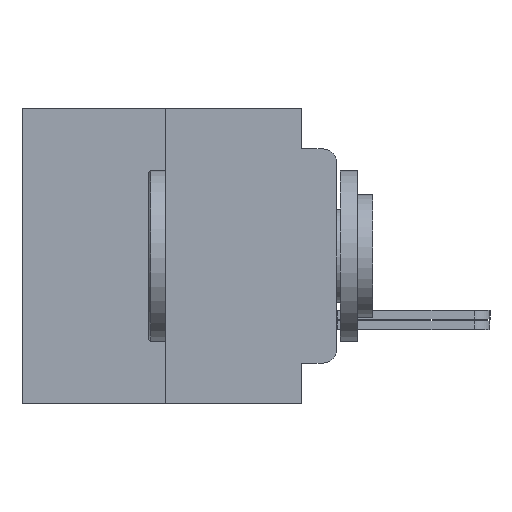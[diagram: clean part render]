
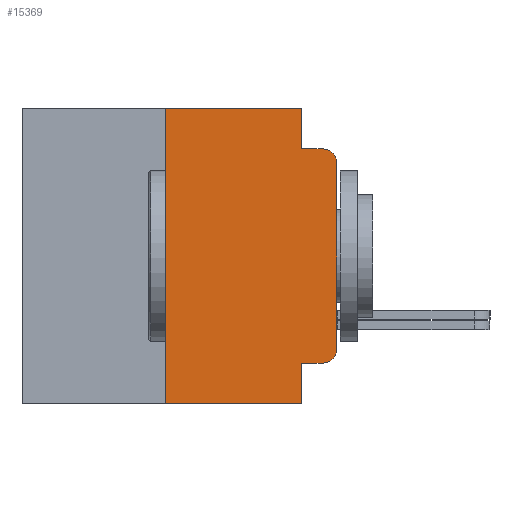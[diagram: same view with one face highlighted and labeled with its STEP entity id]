
A CAD part, left-side view. The second image highlights one B-rep face of the part: STEP entity #15369.
In plain terms, the highlighted planar face has unit normal (-1, 0, 0).
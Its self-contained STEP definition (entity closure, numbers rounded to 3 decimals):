
#266 = VERTEX_POINT ( 'NONE', #17163 ) ;
#475 = PLANE ( 'NONE',  #5160 ) ;
#850 = CARTESIAN_POINT ( 'NONE',  ( -75.603, 11.684, 5.486 ) ) ;
#902 = VERTEX_POINT ( 'NONE', #14047 ) ;
#1233 = DIRECTION ( 'NONE',  ( 0., 0., -1. ) ) ;
#1267 = ORIENTED_EDGE ( 'NONE', *, *, #15515, .F. ) ;
#1921 = VECTOR ( 'NONE', #11337, 1000. ) ;
#2256 = EDGE_CURVE ( 'NONE', #21325, #266, #15595, .T. ) ;
#2447 = CARTESIAN_POINT ( 'NONE',  ( -75.603, 6.35, 5.486 ) ) ;
#2452 = CARTESIAN_POINT ( 'NONE',  ( -75.603, 0.508, 3.467 ) ) ;
#2554 = ORIENTED_EDGE ( 'NONE', *, *, #3513, .T. ) ;
#3513 = EDGE_CURVE ( 'NONE', #18221, #23328, #21067, .T. ) ;
#4085 = CARTESIAN_POINT ( 'NONE',  ( -75.603, 1.295, 3.975 ) ) ;
#4663 = DIRECTION ( 'NONE',  ( -1., 0., 0. ) ) ;
#4794 = CARTESIAN_POINT ( 'NONE',  ( -75.603, 1.295, 0. ) ) ;
#5093 = EDGE_CURVE ( 'NONE', #902, #10016, #17985, .T. ) ;
#5160 = AXIS2_PLACEMENT_3D ( 'NONE', #20195, #9061, #15754 ) ;
#5212 = AXIS2_PLACEMENT_3D ( 'NONE', #2452, #4663, #6886 ) ;
#5741 = ORIENTED_EDGE ( 'NONE', *, *, #27740, .F. ) ;
#6143 = CARTESIAN_POINT ( 'NONE',  ( -75.603, 6.35, -5.486 ) ) ;
#6174 = CIRCLE ( 'NONE', #17892, 0.508 ) ;
#6487 = EDGE_CURVE ( 'NONE', #17211, #7768, #15140, .T. ) ;
#6728 = DIRECTION ( 'NONE',  ( 0., 0., -1. ) ) ;
#6886 = DIRECTION ( 'NONE',  ( 0., 0., -1. ) ) ;
#7120 = DIRECTION ( 'NONE',  ( 0., 0., 1. ) ) ;
#7139 = CARTESIAN_POINT ( 'NONE',  ( -75.603, 6.35, -5.486 ) ) ;
#7324 = ORIENTED_EDGE ( 'NONE', *, *, #2256, .T. ) ;
#7453 = CARTESIAN_POINT ( 'NONE',  ( -75.603, 0.508, -3.467 ) ) ;
#7553 = EDGE_CURVE ( 'NONE', #22178, #902, #11294, .T. ) ;
#7768 = VERTEX_POINT ( 'NONE', #17457 ) ;
#9061 = DIRECTION ( 'NONE',  ( 1., 0., 0. ) ) ;
#9436 = CARTESIAN_POINT ( 'NONE',  ( -75.603, 11.684, -5.486 ) ) ;
#9712 = VECTOR ( 'NONE', #7120, 1000. ) ;
#9891 = VECTOR ( 'NONE', #1233, 1000. ) ;
#10016 = VERTEX_POINT ( 'NONE', #10817 ) ;
#10043 = EDGE_CURVE ( 'NONE', #266, #10016, #17654, .T. ) ;
#10817 = CARTESIAN_POINT ( 'NONE',  ( -75.603, 0.508, 3.975 ) ) ;
#11054 = DIRECTION ( 'NONE',  ( 0., -1., 0. ) ) ;
#11294 = LINE ( 'NONE', #14564, #9891 ) ;
#11337 = DIRECTION ( 'NONE',  ( 0., 0., 1. ) ) ;
#12237 = VECTOR ( 'NONE', #27400, 1000. ) ;
#13430 = VERTEX_POINT ( 'NONE', #2447 ) ;
#13546 = CARTESIAN_POINT ( 'NONE',  ( -75.603, 0., -3.467 ) ) ;
#13614 = ORIENTED_EDGE ( 'NONE', *, *, #10043, .T. ) ;
#14047 = CARTESIAN_POINT ( 'NONE',  ( -75.603, 1.295, 3.975 ) ) ;
#14252 = DIRECTION ( 'NONE',  ( 0., -1., 0. ) ) ;
#14564 = CARTESIAN_POINT ( 'NONE',  ( -75.603, 1.295, 0. ) ) ;
#14803 = VECTOR ( 'NONE', #11054, 1000. ) ;
#14880 = VECTOR ( 'NONE', #26339, 1000. ) ;
#15140 = LINE ( 'NONE', #21773, #14803 ) ;
#15369 = ADVANCED_FACE ( 'NONE', ( #26042 ), #475, .F. ) ;
#15515 = EDGE_CURVE ( 'NONE', #13430, #22178, #21552, .T. ) ;
#15595 = LINE ( 'NONE', #22422, #9712 ) ;
#15754 = DIRECTION ( 'NONE',  ( 0., 0., -1. ) ) ;
#16330 = ORIENTED_EDGE ( 'NONE', *, *, #7553, .F. ) ;
#16786 = CARTESIAN_POINT ( 'NONE',  ( -75.603, 1.295, 5.486 ) ) ;
#17157 = ORIENTED_EDGE ( 'NONE', *, *, #6487, .T. ) ;
#17161 = LINE ( 'NONE', #7139, #1921 ) ;
#17163 = CARTESIAN_POINT ( 'NONE',  ( -75.603, 0., 3.467 ) ) ;
#17211 = VERTEX_POINT ( 'NONE', #18367 ) ;
#17457 = CARTESIAN_POINT ( 'NONE',  ( -75.603, 0.508, -3.975 ) ) ;
#17654 = CIRCLE ( 'NONE', #5212, 0.508 ) ;
#17892 = AXIS2_PLACEMENT_3D ( 'NONE', #7453, #25532, #27744 ) ;
#17985 = LINE ( 'NONE', #4085, #14880 ) ;
#18221 = VERTEX_POINT ( 'NONE', #6143 ) ;
#18367 = CARTESIAN_POINT ( 'NONE',  ( -75.603, 1.295, -3.975 ) ) ;
#20195 = CARTESIAN_POINT ( 'NONE',  ( -75.603, 11.684, 5.486 ) ) ;
#20372 = VECTOR ( 'NONE', #14252, 1000. ) ;
#20597 = CARTESIAN_POINT ( 'NONE',  ( -75.603, 1.295, -5.486 ) ) ;
#21017 = EDGE_CURVE ( 'NONE', #7768, #21325, #6174, .T. ) ;
#21067 = LINE ( 'NONE', #9436, #20372 ) ;
#21325 = VERTEX_POINT ( 'NONE', #13546 ) ;
#21549 = EDGE_LOOP ( 'NONE', ( #17157, #24736, #7324, #13614, #23200, #16330, #1267, #5741, #2554, #25501 ) ) ;
#21552 = LINE ( 'NONE', #850, #12237 ) ;
#21773 = CARTESIAN_POINT ( 'NONE',  ( -75.603, 1.295, -3.975 ) ) ;
#22178 = VERTEX_POINT ( 'NONE', #16786 ) ;
#22422 = CARTESIAN_POINT ( 'NONE',  ( -75.603, 0., 5.486 ) ) ;
#22788 = VECTOR ( 'NONE', #6728, 1000. ) ;
#23200 = ORIENTED_EDGE ( 'NONE', *, *, #5093, .F. ) ;
#23328 = VERTEX_POINT ( 'NONE', #20597 ) ;
#24736 = ORIENTED_EDGE ( 'NONE', *, *, #21017, .T. ) ;
#25501 = ORIENTED_EDGE ( 'NONE', *, *, #26406, .F. ) ;
#25532 = DIRECTION ( 'NONE',  ( -1., 0., 0. ) ) ;
#26042 = FACE_OUTER_BOUND ( 'NONE', #21549, .T. ) ;
#26214 = LINE ( 'NONE', #4794, #22788 ) ;
#26339 = DIRECTION ( 'NONE',  ( 0., -1., 0. ) ) ;
#26406 = EDGE_CURVE ( 'NONE', #17211, #23328, #26214, .T. ) ;
#27400 = DIRECTION ( 'NONE',  ( 0., -1., 0. ) ) ;
#27740 = EDGE_CURVE ( 'NONE', #18221, #13430, #17161, .T. ) ;
#27744 = DIRECTION ( 'NONE',  ( 0., 0., -1. ) ) ;
